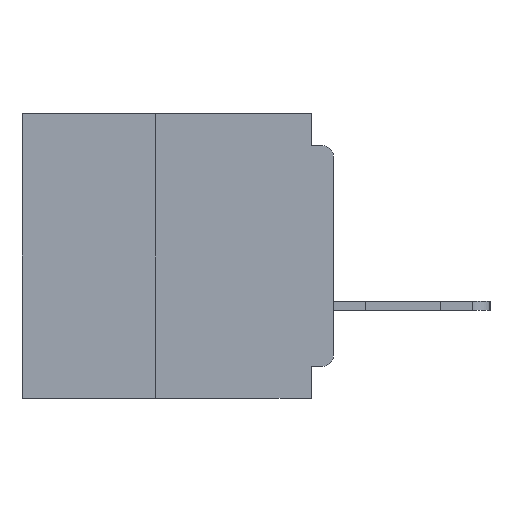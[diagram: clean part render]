
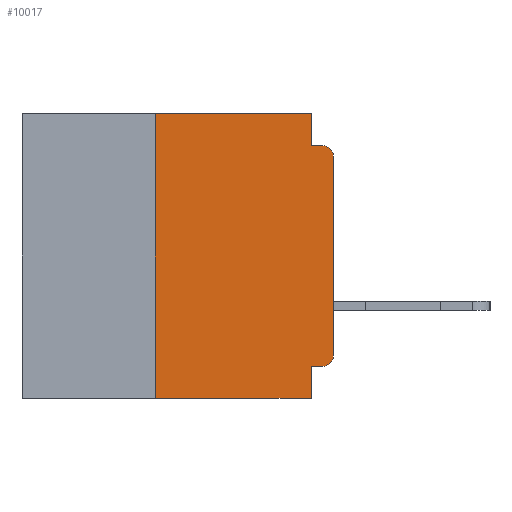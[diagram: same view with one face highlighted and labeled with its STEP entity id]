
A CAD part, left-side view. The second image highlights one B-rep face of the part: STEP entity #10017.
In plain terms, the highlighted planar face has unit normal (-1, 0, 0).
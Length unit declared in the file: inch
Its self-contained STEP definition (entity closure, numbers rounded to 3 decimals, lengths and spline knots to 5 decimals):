
#274 = AXIS2_PLACEMENT_3D ( 'NONE', #18155, #42116, #21584 ) ;
#1837 = EDGE_CURVE ( 'NONE', #43538, #20468, #26293, .T. ) ;
#2032 = CARTESIAN_POINT ( 'NONE',  ( 0., 0.015, -0.045 ) ) ;
#3139 = AXIS2_PLACEMENT_3D ( 'NONE', #26125, #5906, #29687 ) ;
#3746 = EDGE_CURVE ( 'NONE', #34049, #13980, #26645, .T. ) ;
#5313 = DIRECTION ( 'NONE',  ( -1., 0., 0. ) ) ;
#5803 = CARTESIAN_POINT ( 'NONE',  ( 0., 0.031, 0. ) ) ;
#5822 = EDGE_CURVE ( 'NONE', #28677, #22942, #36845, .T. ) ;
#5906 = DIRECTION ( 'NONE',  ( 1., 0., 0. ) ) ;
#6904 = CIRCLE ( 'NONE', #41272, 0.015 ) ;
#7115 = EDGE_CURVE ( 'NONE', #24782, #34072, #37795, .T. ) ;
#9284 = ORIENTED_EDGE ( 'NONE', *, *, #17659, .F. ) ;
#9582 = VECTOR ( 'NONE', #38126, 39.37008 ) ;
#9935 = VECTOR ( 'NONE', #19318, 39.37008 ) ;
#10017 = ADVANCED_FACE ( 'NONE', ( #39649 ), #26276, .F. ) ;
#13980 = VERTEX_POINT ( 'NONE', #35135 ) ;
#15175 = LINE ( 'NONE', #39789, #41415 ) ;
#16199 = ORIENTED_EDGE ( 'NONE', *, *, #41803, .F. ) ;
#16750 = LINE ( 'NONE', #22575, #33864 ) ;
#17659 = EDGE_CURVE ( 'NONE', #13980, #34850, #15175, .T. ) ;
#17931 = LINE ( 'NONE', #26051, #9935 ) ;
#18155 = CARTESIAN_POINT ( 'NONE',  ( 0., 0.015, -0.34 ) ) ;
#18836 = ORIENTED_EDGE ( 'NONE', *, *, #7115, .T. ) ;
#19318 = DIRECTION ( 'NONE',  ( 0., 0., -1. ) ) ;
#19802 = CARTESIAN_POINT ( 'NONE',  ( 0., 0.031, -0.4 ) ) ;
#20123 = ORIENTED_EDGE ( 'NONE', *, *, #28870, .T. ) ;
#20468 = VERTEX_POINT ( 'NONE', #2032 ) ;
#20783 = ORIENTED_EDGE ( 'NONE', *, *, #1837, .F. ) ;
#21584 = DIRECTION ( 'NONE',  ( 0., 0., -1. ) ) ;
#21688 = CARTESIAN_POINT ( 'NONE',  ( 0., 0.015, -0.355 ) ) ;
#22575 = CARTESIAN_POINT ( 'NONE',  ( 0., 0.437, 0. ) ) ;
#22942 = VERTEX_POINT ( 'NONE', #34055 ) ;
#23545 = VECTOR ( 'NONE', #41433, 39.37008 ) ;
#23846 = CARTESIAN_POINT ( 'NONE',  ( 0., 0.25, -0.4 ) ) ;
#24077 = CARTESIAN_POINT ( 'NONE',  ( 0., 0., -0.34 ) ) ;
#24782 = VERTEX_POINT ( 'NONE', #24077 ) ;
#25564 = VECTOR ( 'NONE', #36517, 39.37008 ) ;
#25680 = CARTESIAN_POINT ( 'NONE',  ( 0., 0.015, -0.06 ) ) ;
#26051 = CARTESIAN_POINT ( 'NONE',  ( 0., 0.031, 0. ) ) ;
#26125 = CARTESIAN_POINT ( 'NONE',  ( 0., 0.437, 0. ) ) ;
#26276 = PLANE ( 'NONE',  #3139 ) ;
#26293 = LINE ( 'NONE', #32677, #41326 ) ;
#26319 = ORIENTED_EDGE ( 'NONE', *, *, #3746, .F. ) ;
#26645 = LINE ( 'NONE', #36904, #25564 ) ;
#28636 = VECTOR ( 'NONE', #34644, 39.37008 ) ;
#28677 = VERTEX_POINT ( 'NONE', #23846 ) ;
#28870 = EDGE_CURVE ( 'NONE', #34049, #24782, #34986, .T. ) ;
#29093 = DIRECTION ( 'NONE',  ( 0., 0., -1. ) ) ;
#29419 = DIRECTION ( 'NONE',  ( 0., 0., -1. ) ) ;
#29687 = DIRECTION ( 'NONE',  ( 0., 0., -1. ) ) ;
#31074 = VERTEX_POINT ( 'NONE', #5803 ) ;
#31581 = EDGE_CURVE ( 'NONE', #34072, #20468, #6904, .T. ) ;
#32197 = CARTESIAN_POINT ( 'NONE',  ( 0., 0.031, -0.045 ) ) ;
#32677 = CARTESIAN_POINT ( 'NONE',  ( 0., 0., -0.045 ) ) ;
#32978 = DIRECTION ( 'NONE',  ( 0., -1., 0. ) ) ;
#33864 = VECTOR ( 'NONE', #39800, 39.37008 ) ;
#34049 = VERTEX_POINT ( 'NONE', #21688 ) ;
#34055 = CARTESIAN_POINT ( 'NONE',  ( 0., 0.25, 0. ) ) ;
#34072 = VERTEX_POINT ( 'NONE', #35483 ) ;
#34220 = EDGE_CURVE ( 'NONE', #22942, #31074, #16750, .T. ) ;
#34546 = ORIENTED_EDGE ( 'NONE', *, *, #34220, .F. ) ;
#34644 = DIRECTION ( 'NONE',  ( 0., 0., 1. ) ) ;
#34850 = VERTEX_POINT ( 'NONE', #19802 ) ;
#34986 = CIRCLE ( 'NONE', #274, 0.015 ) ;
#35135 = CARTESIAN_POINT ( 'NONE',  ( 0., 0.031, -0.355 ) ) ;
#35483 = CARTESIAN_POINT ( 'NONE',  ( 0., 0., -0.06 ) ) ;
#35814 = CARTESIAN_POINT ( 'NONE',  ( 0., 0., 0. ) ) ;
#36208 = EDGE_CURVE ( 'NONE', #28677, #34850, #42860, .T. ) ;
#36517 = DIRECTION ( 'NONE',  ( 0., 1., 0. ) ) ;
#36845 = LINE ( 'NONE', #38225, #9582 ) ;
#36904 = CARTESIAN_POINT ( 'NONE',  ( 0., 0., -0.355 ) ) ;
#37264 = ORIENTED_EDGE ( 'NONE', *, *, #31581, .T. ) ;
#37795 = LINE ( 'NONE', #35814, #28636 ) ;
#37988 = CARTESIAN_POINT ( 'NONE',  ( 0., 0.437, -0.4 ) ) ;
#38126 = DIRECTION ( 'NONE',  ( 0., 0., 1. ) ) ;
#38225 = CARTESIAN_POINT ( 'NONE',  ( 0., 0.25, -0.4 ) ) ;
#39649 = FACE_OUTER_BOUND ( 'NONE', #41936, .T. ) ;
#39789 = CARTESIAN_POINT ( 'NONE',  ( 0., 0.031, -0.4 ) ) ;
#39800 = DIRECTION ( 'NONE',  ( 0., -1., 0. ) ) ;
#41272 = AXIS2_PLACEMENT_3D ( 'NONE', #25680, #5313, #29093 ) ;
#41326 = VECTOR ( 'NONE', #32978, 39.37008 ) ;
#41415 = VECTOR ( 'NONE', #29419, 39.37008 ) ;
#41433 = DIRECTION ( 'NONE',  ( 0., -1., 0. ) ) ;
#41803 = EDGE_CURVE ( 'NONE', #31074, #43538, #17931, .T. ) ;
#41936 = EDGE_LOOP ( 'NONE', ( #18836, #37264, #20783, #16199, #34546, #42647, #43638, #9284, #26319, #20123 ) ) ;
#42116 = DIRECTION ( 'NONE',  ( -1., 0., 0. ) ) ;
#42647 = ORIENTED_EDGE ( 'NONE', *, *, #5822, .F. ) ;
#42860 = LINE ( 'NONE', #37988, #23545 ) ;
#43538 = VERTEX_POINT ( 'NONE', #32197 ) ;
#43638 = ORIENTED_EDGE ( 'NONE', *, *, #36208, .T. ) ;
